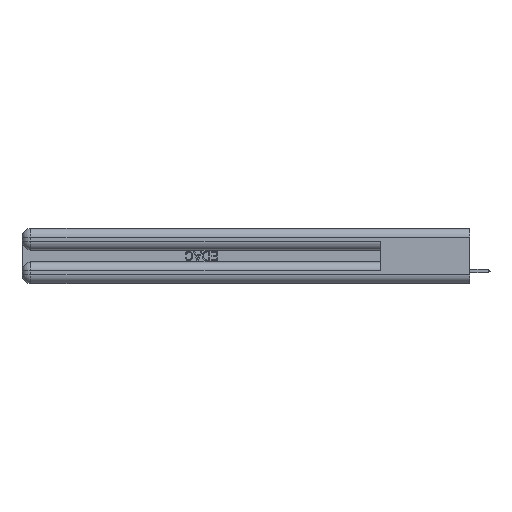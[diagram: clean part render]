
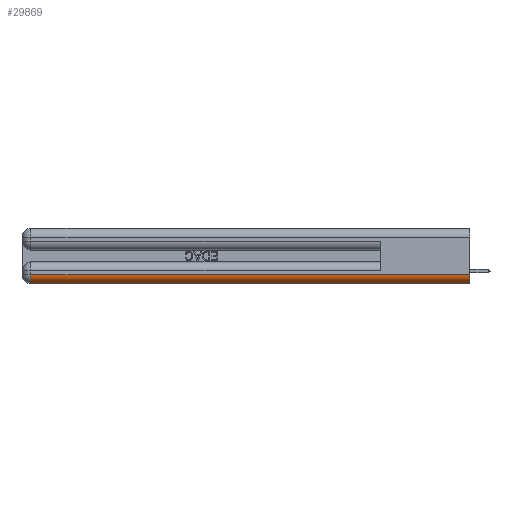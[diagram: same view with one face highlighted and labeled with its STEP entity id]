
A CAD part, left-side view. The second image highlights one B-rep face of the part: STEP entity #29869.
In plain terms, the highlighted cylindrical face has radius 1.524 mm (diameter 3.048 mm), a partial arc.
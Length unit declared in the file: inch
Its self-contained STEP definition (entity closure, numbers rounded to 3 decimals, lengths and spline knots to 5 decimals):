
#1687 = CARTESIAN_POINT ( 'NONE',  ( 0.06, 3., 0. ) ) ;
#4228 = VERTEX_POINT ( 'NONE', #7077 ) ;
#5796 = ORIENTED_EDGE ( 'NONE', *, *, #8025, .F. ) ;
#6344 = FACE_OUTER_BOUND ( 'NONE', #25148, .T. ) ;
#6961 = EDGE_CURVE ( 'NONE', #4228, #41025, #8861, .T. ) ;
#7077 = CARTESIAN_POINT ( 'NONE',  ( 0., 2.94, 0.06 ) ) ;
#8025 = EDGE_CURVE ( 'NONE', #27200, #4228, #41084, .T. ) ;
#8546 = ORIENTED_EDGE ( 'NONE', *, *, #6961, .F. ) ;
#8861 = LINE ( 'NONE', #46262, #17429 ) ;
#11956 = EDGE_CURVE ( 'NONE', #41025, #48609, #22284, .T. ) ;
#12999 = CYLINDRICAL_SURFACE ( 'NONE', #40356, 0.06 ) ;
#13166 = DIRECTION ( 'NONE',  ( 0., 1., 0. ) ) ;
#14369 = DIRECTION ( 'NONE',  ( 0., -1., 0. ) ) ;
#16512 = AXIS2_PLACEMENT_3D ( 'NONE', #19349, #42988, #19505 ) ;
#16676 = DIRECTION ( 'NONE',  ( 0., -1., 0. ) ) ;
#17429 = VECTOR ( 'NONE', #16676, 39.37008 ) ;
#17469 = EDGE_CURVE ( 'NONE', #48609, #27200, #31478, .T. ) ;
#18268 = DIRECTION ( 'NONE',  ( 0., 0., 1. ) ) ;
#19349 = CARTESIAN_POINT ( 'NONE',  ( 0.06, 2.94, 0.06 ) ) ;
#19505 = DIRECTION ( 'NONE',  ( 0., 0., 1. ) ) ;
#21510 = DIRECTION ( 'NONE',  ( 0., 0., 1. ) ) ;
#22284 = CIRCLE ( 'NONE', #25821, 0.06 ) ;
#24533 = DIRECTION ( 'NONE',  ( 0., 1., 0. ) ) ;
#25148 = EDGE_LOOP ( 'NONE', ( #47367, #8546, #5796, #43249 ) ) ;
#25821 = AXIS2_PLACEMENT_3D ( 'NONE', #45151, #14369, #18268 ) ;
#27200 = VERTEX_POINT ( 'NONE', #33284 ) ;
#27288 = CARTESIAN_POINT ( 'NONE',  ( 0., 0., 0.06 ) ) ;
#29869 = ADVANCED_FACE ( 'NONE', ( #6344 ), #12999, .T. ) ;
#31478 = LINE ( 'NONE', #1687, #40617 ) ;
#33284 = CARTESIAN_POINT ( 'NONE',  ( 0.06, 2.94, 0. ) ) ;
#35326 = CARTESIAN_POINT ( 'NONE',  ( 0.06, 0., 0. ) ) ;
#37185 = CARTESIAN_POINT ( 'NONE',  ( 0.06, 0., 0.06 ) ) ;
#40356 = AXIS2_PLACEMENT_3D ( 'NONE', #37185, #24533, #21510 ) ;
#40617 = VECTOR ( 'NONE', #13166, 39.37008 ) ;
#41025 = VERTEX_POINT ( 'NONE', #27288 ) ;
#41084 = CIRCLE ( 'NONE', #16512, 0.06 ) ;
#42988 = DIRECTION ( 'NONE',  ( 0., 1., 0. ) ) ;
#43249 = ORIENTED_EDGE ( 'NONE', *, *, #17469, .F. ) ;
#45151 = CARTESIAN_POINT ( 'NONE',  ( 0.06, 0., 0.06 ) ) ;
#46262 = CARTESIAN_POINT ( 'NONE',  ( 0., 0., 0.06 ) ) ;
#47367 = ORIENTED_EDGE ( 'NONE', *, *, #11956, .F. ) ;
#48609 = VERTEX_POINT ( 'NONE', #35326 ) ;
